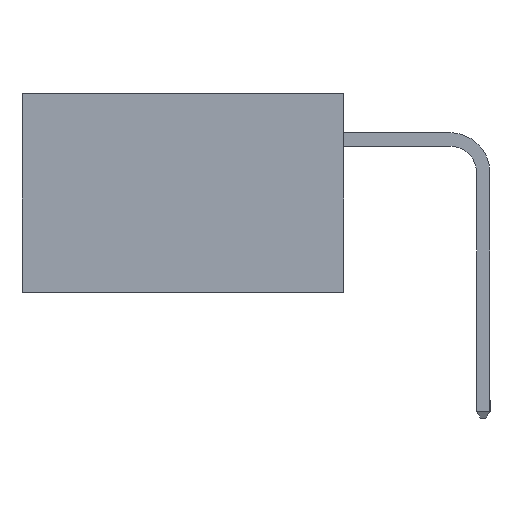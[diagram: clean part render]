
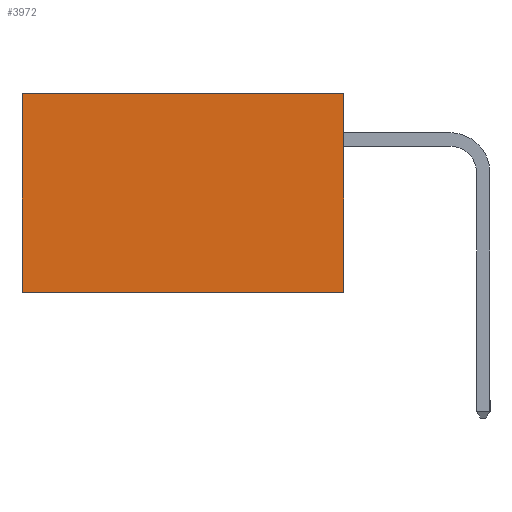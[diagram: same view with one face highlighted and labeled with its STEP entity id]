
A CAD part, left-side view. The second image highlights one B-rep face of the part: STEP entity #3972.
In plain terms, the highlighted planar face has unit normal (-1, 0, 0).
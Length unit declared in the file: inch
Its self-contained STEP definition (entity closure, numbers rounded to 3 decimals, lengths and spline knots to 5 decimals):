
#585 = VECTOR ( 'NONE', #20785, 39.37008 ) ;
#3308 = CARTESIAN_POINT ( 'NONE',  ( 0.2615, 0., -0.37 ) ) ;
#3972 = ADVANCED_FACE ( 'NONE', ( #15135 ), #14911, .F. ) ;
#4912 = CARTESIAN_POINT ( 'NONE',  ( 0.2615, 0.6, 0. ) ) ;
#5253 = DIRECTION ( 'NONE',  ( 0., 0., -1. ) ) ;
#5502 = VERTEX_POINT ( 'NONE', #9625 ) ;
#6821 = VERTEX_POINT ( 'NONE', #4912 ) ;
#7424 = LINE ( 'NONE', #8811, #11376 ) ;
#8151 = EDGE_CURVE ( 'NONE', #6821, #19149, #7424, .T. ) ;
#8811 = CARTESIAN_POINT ( 'NONE',  ( 0.2615, 0.6, -0.37 ) ) ;
#8886 = CARTESIAN_POINT ( 'NONE',  ( 0.2615, 0.6, -0.37 ) ) ;
#9360 = DIRECTION ( 'NONE',  ( 0., 1., 0. ) ) ;
#9625 = CARTESIAN_POINT ( 'NONE',  ( 0.2615, 0., -0.37 ) ) ;
#10741 = AXIS2_PLACEMENT_3D ( 'NONE', #3308, #16877, #5253 ) ;
#10933 = CARTESIAN_POINT ( 'NONE',  ( 0.2615, 0., 0. ) ) ;
#11214 = EDGE_LOOP ( 'NONE', ( #21583, #16979, #12608, #13956 ) ) ;
#11376 = VECTOR ( 'NONE', #24311, 39.37008 ) ;
#12608 = ORIENTED_EDGE ( 'NONE', *, *, #13352, .F. ) ;
#13352 = EDGE_CURVE ( 'NONE', #14354, #5502, #24163, .T. ) ;
#13834 = CARTESIAN_POINT ( 'NONE',  ( 0.2615, 0., -0.37 ) ) ;
#13956 = ORIENTED_EDGE ( 'NONE', *, *, #16185, .T. ) ;
#14354 = VERTEX_POINT ( 'NONE', #10933 ) ;
#14911 = PLANE ( 'NONE',  #10741 ) ;
#15135 = FACE_OUTER_BOUND ( 'NONE', #11214, .T. ) ;
#15274 = LINE ( 'NONE', #19013, #24963 ) ;
#15804 = DIRECTION ( 'NONE',  ( 0., 0., -1. ) ) ;
#16185 = EDGE_CURVE ( 'NONE', #14354, #6821, #15274, .T. ) ;
#16648 = LINE ( 'NONE', #24583, #585 ) ;
#16877 = DIRECTION ( 'NONE',  ( 1., 0., 0. ) ) ;
#16979 = ORIENTED_EDGE ( 'NONE', *, *, #20412, .F. ) ;
#19013 = CARTESIAN_POINT ( 'NONE',  ( 0.2615, 0., 0. ) ) ;
#19149 = VERTEX_POINT ( 'NONE', #8886 ) ;
#20412 = EDGE_CURVE ( 'NONE', #5502, #19149, #16648, .T. ) ;
#20785 = DIRECTION ( 'NONE',  ( 0., 1., 0. ) ) ;
#21583 = ORIENTED_EDGE ( 'NONE', *, *, #8151, .T. ) ;
#23559 = VECTOR ( 'NONE', #15804, 39.37008 ) ;
#24163 = LINE ( 'NONE', #13834, #23559 ) ;
#24311 = DIRECTION ( 'NONE',  ( 0., 0., -1. ) ) ;
#24583 = CARTESIAN_POINT ( 'NONE',  ( 0.2615, 0., -0.37 ) ) ;
#24963 = VECTOR ( 'NONE', #9360, 39.37008 ) ;
